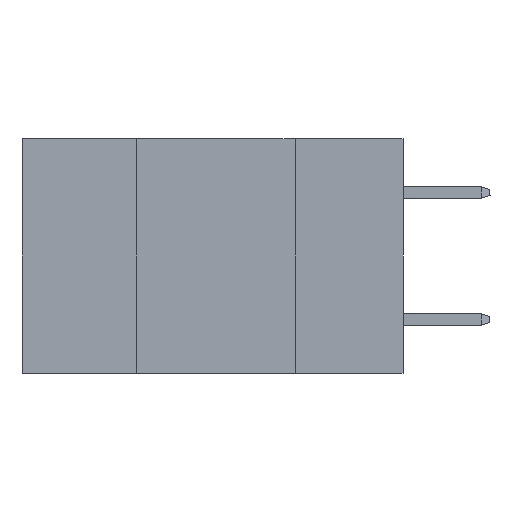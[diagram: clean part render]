
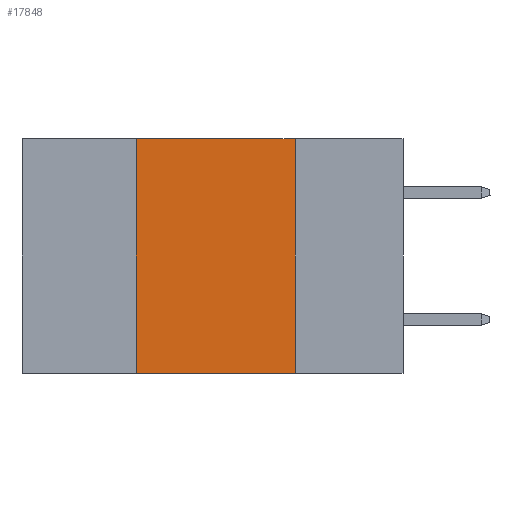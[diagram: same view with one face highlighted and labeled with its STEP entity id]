
A CAD part, left-side view. The second image highlights one B-rep face of the part: STEP entity #17848.
In plain terms, the highlighted planar face has unit normal (-1, 0, 0).
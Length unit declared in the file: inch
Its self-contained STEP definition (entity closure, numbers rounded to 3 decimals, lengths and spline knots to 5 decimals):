
#194 = LINE ( 'NONE', #4637, #14488 ) ;
#509 = VECTOR ( 'NONE', #8329, 39.37008 ) ;
#842 = CARTESIAN_POINT ( 'NONE',  ( 0., 0.17, 0. ) ) ;
#1267 = EDGE_CURVE ( 'NONE', #11269, #6676, #6362, .T. ) ;
#1839 = CARTESIAN_POINT ( 'NONE',  ( 0., 0.6, 0. ) ) ;
#2111 = DIRECTION ( 'NONE',  ( 1., 0., 0. ) ) ;
#2459 = DIRECTION ( 'NONE',  ( 0., 0., 1. ) ) ;
#4020 = VECTOR ( 'NONE', #14616, 39.37008 ) ;
#4637 = CARTESIAN_POINT ( 'NONE',  ( 0., 0.17, 0. ) ) ;
#5882 = EDGE_CURVE ( 'NONE', #19718, #13705, #14740, .T. ) ;
#6029 = CARTESIAN_POINT ( 'NONE',  ( 0., 0.6, 0. ) ) ;
#6362 = LINE ( 'NONE', #17953, #4020 ) ;
#6448 = FACE_OUTER_BOUND ( 'NONE', #20709, .T. ) ;
#6676 = VERTEX_POINT ( 'NONE', #11506 ) ;
#8171 = DIRECTION ( 'NONE',  ( 0., 0., -1. ) ) ;
#8329 = DIRECTION ( 'NONE',  ( 0., -1., 0. ) ) ;
#8749 = CARTESIAN_POINT ( 'NONE',  ( 0., 0.42, 0. ) ) ;
#8786 = ORIENTED_EDGE ( 'NONE', *, *, #5882, .F. ) ;
#9642 = CARTESIAN_POINT ( 'NONE',  ( 0., 0.42, -0.37 ) ) ;
#11269 = VERTEX_POINT ( 'NONE', #9642 ) ;
#11506 = CARTESIAN_POINT ( 'NONE',  ( 0., 0.17, -0.37 ) ) ;
#13705 = VERTEX_POINT ( 'NONE', #842 ) ;
#14488 = VECTOR ( 'NONE', #8171, 39.37008 ) ;
#14616 = DIRECTION ( 'NONE',  ( 0., -1., 0. ) ) ;
#14643 = EDGE_CURVE ( 'NONE', #13705, #6676, #194, .T. ) ;
#14740 = LINE ( 'NONE', #1839, #509 ) ;
#15104 = CARTESIAN_POINT ( 'NONE',  ( 0., 0.42, 0. ) ) ;
#15644 = PLANE ( 'NONE',  #18525 ) ;
#15773 = EDGE_CURVE ( 'NONE', #11269, #19718, #16936, .T. ) ;
#16090 = ORIENTED_EDGE ( 'NONE', *, *, #1267, .T. ) ;
#16558 = VECTOR ( 'NONE', #2459, 39.37008 ) ;
#16936 = LINE ( 'NONE', #8749, #16558 ) ;
#17556 = ORIENTED_EDGE ( 'NONE', *, *, #14643, .F. ) ;
#17848 = ADVANCED_FACE ( 'NONE', ( #6448 ), #15644, .F. ) ;
#17953 = CARTESIAN_POINT ( 'NONE',  ( 0., 0.6, -0.37 ) ) ;
#18525 = AXIS2_PLACEMENT_3D ( 'NONE', #6029, #2111, #19708 ) ;
#19133 = ORIENTED_EDGE ( 'NONE', *, *, #15773, .F. ) ;
#19708 = DIRECTION ( 'NONE',  ( 0., 0., -1. ) ) ;
#19718 = VERTEX_POINT ( 'NONE', #15104 ) ;
#20709 = EDGE_LOOP ( 'NONE', ( #17556, #8786, #19133, #16090 ) ) ;
